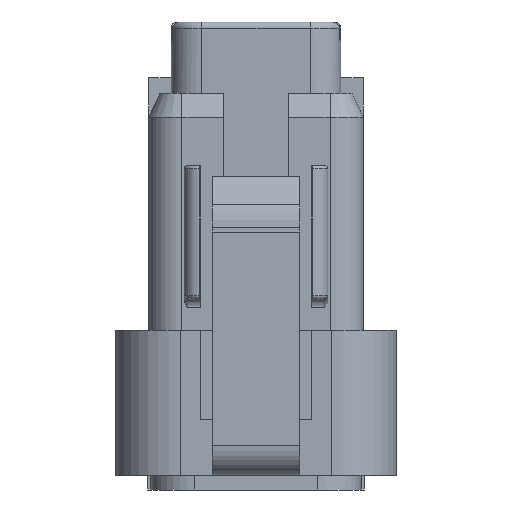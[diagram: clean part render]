
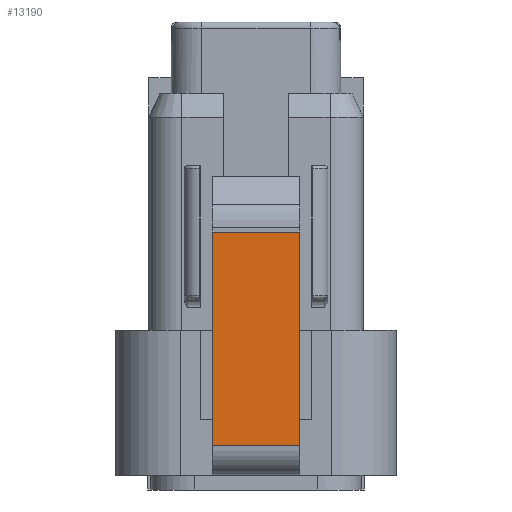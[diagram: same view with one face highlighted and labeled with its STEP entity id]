
A CAD part, front view. The second image highlights one B-rep face of the part: STEP entity #13190.
In plain terms, the highlighted face is planar.
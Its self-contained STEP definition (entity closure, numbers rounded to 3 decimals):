
#444 = DIRECTION ( 'NONE',  ( 0., 1., 0. ) ) ;
#1521 = DIRECTION ( 'NONE',  ( 0., 1., 0. ) ) ;
#1943 = CARTESIAN_POINT ( 'NONE',  ( -1.45, 17.4, 5.325 ) ) ;
#2619 = EDGE_CURVE ( 'NONE', #13780, #3571, #19334, .T. ) ;
#3571 = VERTEX_POINT ( 'NONE', #13801 ) ;
#4026 = CARTESIAN_POINT ( 'NONE',  ( 1.45, 10.25, 5.325 ) ) ;
#4995 = VECTOR ( 'NONE', #1521, 1000. ) ;
#5640 = VECTOR ( 'NONE', #8160, 1000. ) ;
#5978 = EDGE_CURVE ( 'NONE', #3571, #10998, #16466, .T. ) ;
#7033 = CARTESIAN_POINT ( 'NONE',  ( -1.45, 10.25, 5.325 ) ) ;
#7460 = VECTOR ( 'NONE', #11275, 1000. ) ;
#7899 = LINE ( 'NONE', #12581, #4995 ) ;
#8160 = DIRECTION ( 'NONE',  ( -1., 0., 0. ) ) ;
#8589 = LINE ( 'NONE', #10193, #5640 ) ;
#8951 = CARTESIAN_POINT ( 'NONE',  ( 1.45, 17.4, 5.325 ) ) ;
#8953 = VECTOR ( 'NONE', #444, 1000. ) ;
#9248 = ORIENTED_EDGE ( 'NONE', *, *, #11424, .T. ) ;
#9471 = CARTESIAN_POINT ( 'NONE',  ( 1.45, 10.25, 5.325 ) ) ;
#9871 = ORIENTED_EDGE ( 'NONE', *, *, #2619, .F. ) ;
#10001 = PLANE ( 'NONE',  #15113 ) ;
#10193 = CARTESIAN_POINT ( 'NONE',  ( 1.45, 17.4, 5.325 ) ) ;
#10347 = EDGE_LOOP ( 'NONE', ( #16083, #11471, #9871, #9248 ) ) ;
#10998 = VERTEX_POINT ( 'NONE', #1943 ) ;
#11275 = DIRECTION ( 'NONE',  ( -1., 0., 0. ) ) ;
#11424 = EDGE_CURVE ( 'NONE', #13780, #20207, #7899, .T. ) ;
#11471 = ORIENTED_EDGE ( 'NONE', *, *, #5978, .F. ) ;
#12581 = CARTESIAN_POINT ( 'NONE',  ( 1.45, 10.25, 5.325 ) ) ;
#13190 = ADVANCED_FACE ( 'NONE', ( #19764 ), #10001, .T. ) ;
#13522 = DIRECTION ( 'NONE',  ( 0., 1., 0. ) ) ;
#13654 = EDGE_CURVE ( 'NONE', #20207, #10998, #8589, .T. ) ;
#13780 = VERTEX_POINT ( 'NONE', #4026 ) ;
#13801 = CARTESIAN_POINT ( 'NONE',  ( -1.45, 10.25, 5.325 ) ) ;
#14985 = CARTESIAN_POINT ( 'NONE',  ( 1.45, 10.25, 5.325 ) ) ;
#15113 = AXIS2_PLACEMENT_3D ( 'NONE', #14985, #19662, #13522 ) ;
#16083 = ORIENTED_EDGE ( 'NONE', *, *, #13654, .T. ) ;
#16466 = LINE ( 'NONE', #7033, #8953 ) ;
#19334 = LINE ( 'NONE', #9471, #7460 ) ;
#19662 = DIRECTION ( 'NONE',  ( 0., 0., 1. ) ) ;
#19764 = FACE_OUTER_BOUND ( 'NONE', #10347, .T. ) ;
#20207 = VERTEX_POINT ( 'NONE', #8951 ) ;
